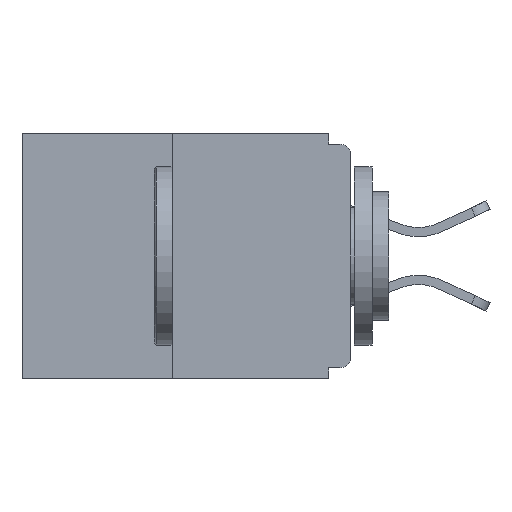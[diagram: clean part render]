
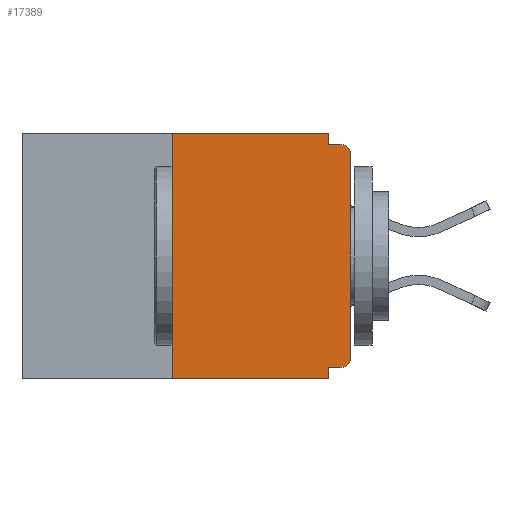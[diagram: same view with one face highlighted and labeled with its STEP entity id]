
A CAD part, left-side view. The second image highlights one B-rep face of the part: STEP entity #17389.
In plain terms, the highlighted planar face has unit normal (-1, 0, 0).
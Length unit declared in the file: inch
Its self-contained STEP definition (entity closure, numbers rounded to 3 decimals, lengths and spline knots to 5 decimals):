
#133 = EDGE_CURVE ( 'NONE', #17221, #15312, #7931, .T. ) ;
#461 = ORIENTED_EDGE ( 'NONE', *, *, #22560, .T. ) ;
#1425 = LINE ( 'NONE', #9230, #18892 ) ;
#1450 = LINE ( 'NONE', #4006, #11769 ) ;
#1636 = VERTEX_POINT ( 'NONE', #16660 ) ;
#1707 = LINE ( 'NONE', #14552, #20615 ) ;
#2205 = CARTESIAN_POINT ( 'NONE',  ( 0., 0.25, -0.343 ) ) ;
#2408 = CARTESIAN_POINT ( 'NONE',  ( 0., 0.031, -0.015 ) ) ;
#2725 = ORIENTED_EDGE ( 'NONE', *, *, #5386, .T. ) ;
#3331 = CARTESIAN_POINT ( 'NONE',  ( 0., 0.46, 0. ) ) ;
#3707 = EDGE_CURVE ( 'NONE', #8989, #19070, #16350, .T. ) ;
#3794 = EDGE_LOOP ( 'NONE', ( #16299, #11242, #10285, #11839, #18101, #461, #2725, #16093, #22406, #6519 ) ) ;
#3865 = CARTESIAN_POINT ( 'NONE',  ( 0., 0.46, -0.343 ) ) ;
#4003 = EDGE_CURVE ( 'NONE', #10733, #19070, #1425, .T. ) ;
#4006 = CARTESIAN_POINT ( 'NONE',  ( 0., 0., 0. ) ) ;
#4081 = DIRECTION ( 'NONE',  ( 0., 0., 1. ) ) ;
#5386 = EDGE_CURVE ( 'NONE', #23476, #8989, #1450, .T. ) ;
#5400 = DIRECTION ( 'NONE',  ( 0., -1., 0. ) ) ;
#6519 = ORIENTED_EDGE ( 'NONE', *, *, #19152, .F. ) ;
#6523 = DIRECTION ( 'NONE',  ( 0., 0., -1. ) ) ;
#6794 = CARTESIAN_POINT ( 'NONE',  ( 0., 0.25, 0. ) ) ;
#6815 = DIRECTION ( 'NONE',  ( 0., 0., -1. ) ) ;
#6953 = FACE_OUTER_BOUND ( 'NONE', #3794, .T. ) ;
#6991 = VECTOR ( 'NONE', #21192, 39.37008 ) ;
#7115 = CARTESIAN_POINT ( 'NONE',  ( 0., 0.031, 0. ) ) ;
#7145 = VECTOR ( 'NONE', #11825, 39.37008 ) ;
#7768 = VERTEX_POINT ( 'NONE', #11207 ) ;
#7821 = VERTEX_POINT ( 'NONE', #9456 ) ;
#7931 = LINE ( 'NONE', #3865, #9929 ) ;
#8279 = DIRECTION ( 'NONE',  ( -1., 0., 0. ) ) ;
#8420 = PLANE ( 'NONE',  #16932 ) ;
#8673 = VECTOR ( 'NONE', #21391, 39.37008 ) ;
#8989 = VERTEX_POINT ( 'NONE', #22618 ) ;
#9230 = CARTESIAN_POINT ( 'NONE',  ( 0., 0., -0.015 ) ) ;
#9442 = LINE ( 'NONE', #15252, #7145 ) ;
#9456 = CARTESIAN_POINT ( 'NONE',  ( 0., 0.25, 0. ) ) ;
#9606 = CIRCLE ( 'NONE', #17754, 0.015 ) ;
#9658 = EDGE_CURVE ( 'NONE', #17221, #7821, #18437, .T. ) ;
#9789 = LINE ( 'NONE', #7115, #10621 ) ;
#9929 = VECTOR ( 'NONE', #12875, 39.37008 ) ;
#10285 = ORIENTED_EDGE ( 'NONE', *, *, #133, .T. ) ;
#10621 = VECTOR ( 'NONE', #23392, 39.37008 ) ;
#10733 = VERTEX_POINT ( 'NONE', #2408 ) ;
#11207 = CARTESIAN_POINT ( 'NONE',  ( 0., 0.015, -0.328 ) ) ;
#11242 = ORIENTED_EDGE ( 'NONE', *, *, #9658, .F. ) ;
#11769 = VECTOR ( 'NONE', #4081, 39.37008 ) ;
#11825 = DIRECTION ( 'NONE',  ( 0., 0., -1. ) ) ;
#11839 = ORIENTED_EDGE ( 'NONE', *, *, #14026, .F. ) ;
#12875 = DIRECTION ( 'NONE',  ( 0., -1., 0. ) ) ;
#12878 = CARTESIAN_POINT ( 'NONE',  ( 0., 0.031, -0.328 ) ) ;
#13218 = CARTESIAN_POINT ( 'NONE',  ( 0., 0.031, -0.343 ) ) ;
#13444 = DIRECTION ( 'NONE',  ( -1., 0., 0. ) ) ;
#14026 = EDGE_CURVE ( 'NONE', #22275, #15312, #9442, .T. ) ;
#14091 = LINE ( 'NONE', #3331, #8673 ) ;
#14552 = CARTESIAN_POINT ( 'NONE',  ( 0., 0., -0.328 ) ) ;
#14682 = CARTESIAN_POINT ( 'NONE',  ( 0., 0., -0.313 ) ) ;
#15252 = CARTESIAN_POINT ( 'NONE',  ( 0., 0.031, -0.343 ) ) ;
#15256 = DIRECTION ( 'NONE',  ( 0., 0., -1. ) ) ;
#15312 = VERTEX_POINT ( 'NONE', #13218 ) ;
#15566 = CARTESIAN_POINT ( 'NONE',  ( 0., 0.015, -0.313 ) ) ;
#16093 = ORIENTED_EDGE ( 'NONE', *, *, #3707, .T. ) ;
#16162 = DIRECTION ( 'NONE',  ( 0., 1., 0. ) ) ;
#16299 = ORIENTED_EDGE ( 'NONE', *, *, #18655, .F. ) ;
#16350 = CIRCLE ( 'NONE', #20382, 0.015 ) ;
#16660 = CARTESIAN_POINT ( 'NONE',  ( 0., 0.031, 0. ) ) ;
#16932 = AXIS2_PLACEMENT_3D ( 'NONE', #21358, #21212, #6815 ) ;
#17221 = VERTEX_POINT ( 'NONE', #2205 ) ;
#17389 = ADVANCED_FACE ( 'NONE', ( #6953 ), #8420, .F. ) ;
#17502 = CARTESIAN_POINT ( 'NONE',  ( 0., 0.015, -0.015 ) ) ;
#17754 = AXIS2_PLACEMENT_3D ( 'NONE', #15566, #13444, #15256 ) ;
#18101 = ORIENTED_EDGE ( 'NONE', *, *, #20016, .F. ) ;
#18437 = LINE ( 'NONE', #6794, #6991 ) ;
#18655 = EDGE_CURVE ( 'NONE', #7821, #1636, #14091, .T. ) ;
#18892 = VECTOR ( 'NONE', #5400, 39.37008 ) ;
#19070 = VERTEX_POINT ( 'NONE', #17502 ) ;
#19152 = EDGE_CURVE ( 'NONE', #1636, #10733, #9789, .T. ) ;
#20016 = EDGE_CURVE ( 'NONE', #7768, #22275, #1707, .T. ) ;
#20382 = AXIS2_PLACEMENT_3D ( 'NONE', #21289, #8279, #6523 ) ;
#20615 = VECTOR ( 'NONE', #16162, 39.37008 ) ;
#21192 = DIRECTION ( 'NONE',  ( 0., 0., 1. ) ) ;
#21212 = DIRECTION ( 'NONE',  ( 1., 0., 0. ) ) ;
#21289 = CARTESIAN_POINT ( 'NONE',  ( 0., 0.015, -0.03 ) ) ;
#21358 = CARTESIAN_POINT ( 'NONE',  ( 0., 0.46, 0. ) ) ;
#21391 = DIRECTION ( 'NONE',  ( 0., -1., 0. ) ) ;
#22275 = VERTEX_POINT ( 'NONE', #12878 ) ;
#22406 = ORIENTED_EDGE ( 'NONE', *, *, #4003, .F. ) ;
#22560 = EDGE_CURVE ( 'NONE', #7768, #23476, #9606, .T. ) ;
#22618 = CARTESIAN_POINT ( 'NONE',  ( 0., 0., -0.03 ) ) ;
#23392 = DIRECTION ( 'NONE',  ( 0., 0., -1. ) ) ;
#23476 = VERTEX_POINT ( 'NONE', #14682 ) ;
